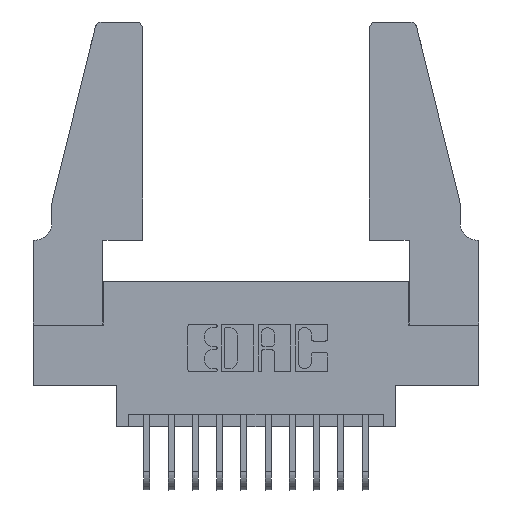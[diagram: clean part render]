
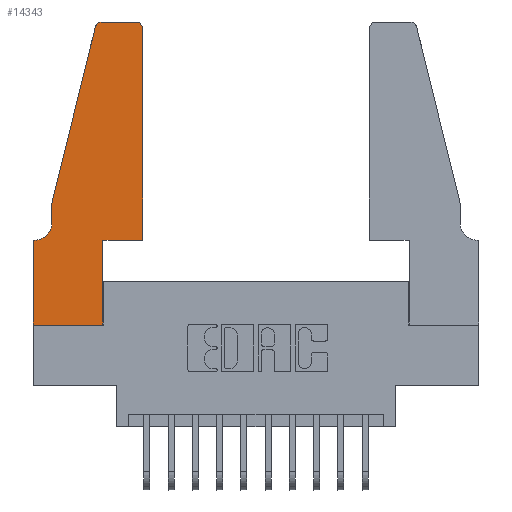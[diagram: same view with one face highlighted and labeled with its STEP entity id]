
A CAD part, top view. The second image highlights one B-rep face of the part: STEP entity #14343.
In plain terms, the highlighted planar face has unit normal (0, 0, 1).
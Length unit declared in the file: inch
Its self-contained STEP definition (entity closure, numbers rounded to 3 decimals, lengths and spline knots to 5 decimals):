
#37 = EDGE_CURVE ( 'NONE', #7963, #10029, #10249, .T. ) ;
#86 = EDGE_CURVE ( 'NONE', #5072, #12838, #6253, .T. ) ;
#127 = EDGE_CURVE ( 'NONE', #12838, #8047, #13153, .T. ) ;
#292 = EDGE_CURVE ( 'NONE', #10029, #13268, #3900, .T. ) ;
#404 = ORIENTED_EDGE ( 'NONE', *, *, #1071, .T. ) ;
#696 = DIRECTION ( 'NONE',  ( -0.239, -0.971, 0. ) ) ;
#711 = CARTESIAN_POINT ( 'NONE',  ( 0., 0.35, 0.37 ) ) ;
#833 = VERTEX_POINT ( 'NONE', #10416 ) ;
#957 = FACE_OUTER_BOUND ( 'NONE', #5830, .T. ) ;
#1071 = EDGE_CURVE ( 'NONE', #15226, #11632, #3088, .T. ) ;
#1086 = AXIS2_PLACEMENT_3D ( 'NONE', #13147, #5798, #14364 ) ;
#1293 = DIRECTION ( 'NONE',  ( 0., 1., 0. ) ) ;
#1337 = ORIENTED_EDGE ( 'NONE', *, *, #11416, .T. ) ;
#1415 = AXIS2_PLACEMENT_3D ( 'NONE', #711, #9407, #2057 ) ;
#1574 = VERTEX_POINT ( 'NONE', #4041 ) ;
#1608 = DIRECTION ( 'NONE',  ( -1., 0., 0. ) ) ;
#1734 = ORIENTED_EDGE ( 'NONE', *, *, #14655, .T. ) ;
#1894 = ORIENTED_EDGE ( 'NONE', *, *, #14117, .T. ) ;
#2057 = DIRECTION ( 'NONE',  ( 1., 0., 0. ) ) ;
#2082 = CARTESIAN_POINT ( 'NONE',  ( 0.0055, 0.35, 0.37 ) ) ;
#2097 = LINE ( 'NONE', #14426, #8632 ) ;
#2214 = CIRCLE ( 'NONE', #1086, 0.03 ) ;
#2235 = CARTESIAN_POINT ( 'NONE',  ( 0., 0., 0.37 ) ) ;
#2258 = DIRECTION ( 'NONE',  ( 1., 0., 0. ) ) ;
#2306 = CARTESIAN_POINT ( 'NONE',  ( 0.0755, 0.35, 0.37 ) ) ;
#2670 = ORIENTED_EDGE ( 'NONE', *, *, #12141, .T. ) ;
#2951 = CARTESIAN_POINT ( 'NONE',  ( 0.25487, 1.22718, 0.37 ) ) ;
#2969 = LINE ( 'NONE', #14914, #15260 ) ;
#3088 = LINE ( 'NONE', #2235, #8820 ) ;
#3347 = CARTESIAN_POINT ( 'NONE',  ( 0.2605, 1.25, 0.37 ) ) ;
#3507 = CARTESIAN_POINT ( 'NONE',  ( 0.4505, 0.35, 0.37 ) ) ;
#3552 = EDGE_CURVE ( 'NONE', #1574, #7292, #4745, .T. ) ;
#3603 = VECTOR ( 'NONE', #7777, 39.37008 ) ;
#3630 = EDGE_CURVE ( 'NONE', #8047, #15226, #13004, .T. ) ;
#3696 = DIRECTION ( 'NONE',  ( -1., 0., 0. ) ) ;
#3785 = DIRECTION ( 'NONE',  ( 0., 0., -1. ) ) ;
#3837 = CARTESIAN_POINT ( 'NONE',  ( 0.4505, 0.35, 0.37 ) ) ;
#3900 = CIRCLE ( 'NONE', #15134, 0.03 ) ;
#4041 = CARTESIAN_POINT ( 'NONE',  ( 0.2865, 0.35, 0.37 ) ) ;
#4115 = ORIENTED_EDGE ( 'NONE', *, *, #37, .T. ) ;
#4119 = CARTESIAN_POINT ( 'NONE',  ( 0.2865, 0.35, 0.37 ) ) ;
#4133 = VECTOR ( 'NONE', #696, 39.37008 ) ;
#4223 = DIRECTION ( 'NONE',  ( -1., 0., 0. ) ) ;
#4322 = ORIENTED_EDGE ( 'NONE', *, *, #292, .T. ) ;
#4581 = ORIENTED_EDGE ( 'NONE', *, *, #3552, .T. ) ;
#4745 = LINE ( 'NONE', #3507, #14536 ) ;
#5029 = ORIENTED_EDGE ( 'NONE', *, *, #86, .T. ) ;
#5072 = VERTEX_POINT ( 'NONE', #7804 ) ;
#5119 = DIRECTION ( 'NONE',  ( 0., -1., 0. ) ) ;
#5386 = CARTESIAN_POINT ( 'NONE',  ( 0.0055, 0.42, 0.37 ) ) ;
#5798 = DIRECTION ( 'NONE',  ( 0., 0., 1. ) ) ;
#5830 = EDGE_LOOP ( 'NONE', ( #4115, #4322, #1894, #9196, #5029, #11651, #6489, #404, #1337, #4581, #1734, #2670 ) ) ;
#6132 = AXIS2_PLACEMENT_3D ( 'NONE', #5386, #3785, #4223 ) ;
#6253 = CIRCLE ( 'NONE', #6132, 0.07 ) ;
#6489 = ORIENTED_EDGE ( 'NONE', *, *, #3630, .T. ) ;
#6941 = VERTEX_POINT ( 'NONE', #15444 ) ;
#7033 = EDGE_CURVE ( 'NONE', #833, #5072, #2097, .T. ) ;
#7292 = VERTEX_POINT ( 'NONE', #3837 ) ;
#7427 = LINE ( 'NONE', #8178, #4133 ) ;
#7777 = DIRECTION ( 'NONE',  ( 0., 1., 0. ) ) ;
#7804 = CARTESIAN_POINT ( 'NONE',  ( 0.0755, 0.42, 0.37 ) ) ;
#7963 = VERTEX_POINT ( 'NONE', #14988 ) ;
#8047 = VERTEX_POINT ( 'NONE', #8982 ) ;
#8178 = CARTESIAN_POINT ( 'NONE',  ( 0.0755, 0.5, 0.37 ) ) ;
#8194 = PLANE ( 'NONE',  #1415 ) ;
#8489 = CARTESIAN_POINT ( 'NONE',  ( 0., 0., 0.37 ) ) ;
#8632 = VECTOR ( 'NONE', #15654, 39.37008 ) ;
#8820 = VECTOR ( 'NONE', #10607, 39.37008 ) ;
#8982 = CARTESIAN_POINT ( 'NONE',  ( 0., 0.35, 0.37 ) ) ;
#9196 = ORIENTED_EDGE ( 'NONE', *, *, #7033, .T. ) ;
#9407 = DIRECTION ( 'NONE',  ( 0., 0., 1. ) ) ;
#9708 = VECTOR ( 'NONE', #5119, 39.37008 ) ;
#9865 = VECTOR ( 'NONE', #1608, 39.37008 ) ;
#10029 = VERTEX_POINT ( 'NONE', #14799 ) ;
#10249 = LINE ( 'NONE', #3347, #9865 ) ;
#10416 = CARTESIAN_POINT ( 'NONE',  ( 0.0755, 0.5, 0.37 ) ) ;
#10607 = DIRECTION ( 'NONE',  ( 1., 0., 0. ) ) ;
#11416 = EDGE_CURVE ( 'NONE', #11632, #1574, #15502, .T. ) ;
#11632 = VERTEX_POINT ( 'NONE', #15556 ) ;
#11651 = ORIENTED_EDGE ( 'NONE', *, *, #127, .T. ) ;
#12141 = EDGE_CURVE ( 'NONE', #6941, #7963, #2214, .T. ) ;
#12167 = DIRECTION ( 'NONE',  ( 1., 0., 0. ) ) ;
#12199 = DIRECTION ( 'NONE',  ( 0., 0., 1. ) ) ;
#12268 = CARTESIAN_POINT ( 'NONE',  ( 0.284, 1.22, 0.37 ) ) ;
#12838 = VERTEX_POINT ( 'NONE', #2082 ) ;
#13004 = LINE ( 'NONE', #8489, #9708 ) ;
#13147 = CARTESIAN_POINT ( 'NONE',  ( 0.4205, 1.22, 0.37 ) ) ;
#13153 = LINE ( 'NONE', #2306, #15239 ) ;
#13268 = VERTEX_POINT ( 'NONE', #2951 ) ;
#14117 = EDGE_CURVE ( 'NONE', #13268, #833, #7427, .T. ) ;
#14343 = ADVANCED_FACE ( 'NONE', ( #957 ), #8194, .T. ) ;
#14364 = DIRECTION ( 'NONE',  ( 1., 0., 0. ) ) ;
#14426 = CARTESIAN_POINT ( 'NONE',  ( 0.0755, 0.5, 0.37 ) ) ;
#14536 = VECTOR ( 'NONE', #2258, 39.37008 ) ;
#14655 = EDGE_CURVE ( 'NONE', #7292, #6941, #2969, .T. ) ;
#14788 = CARTESIAN_POINT ( 'NONE',  ( 0., 0., 0.37 ) ) ;
#14799 = CARTESIAN_POINT ( 'NONE',  ( 0.284, 1.25, 0.37 ) ) ;
#14914 = CARTESIAN_POINT ( 'NONE',  ( 0.4505, 0.35, 0.37 ) ) ;
#14988 = CARTESIAN_POINT ( 'NONE',  ( 0.4205, 1.25, 0.37 ) ) ;
#15134 = AXIS2_PLACEMENT_3D ( 'NONE', #12268, #12199, #12167 ) ;
#15226 = VERTEX_POINT ( 'NONE', #14788 ) ;
#15239 = VECTOR ( 'NONE', #3696, 39.37008 ) ;
#15260 = VECTOR ( 'NONE', #1293, 39.37008 ) ;
#15444 = CARTESIAN_POINT ( 'NONE',  ( 0.4505, 1.22, 0.37 ) ) ;
#15502 = LINE ( 'NONE', #4119, #3603 ) ;
#15556 = CARTESIAN_POINT ( 'NONE',  ( 0.2865, 0., 0.37 ) ) ;
#15654 = DIRECTION ( 'NONE',  ( 0., -1., 0. ) ) ;
